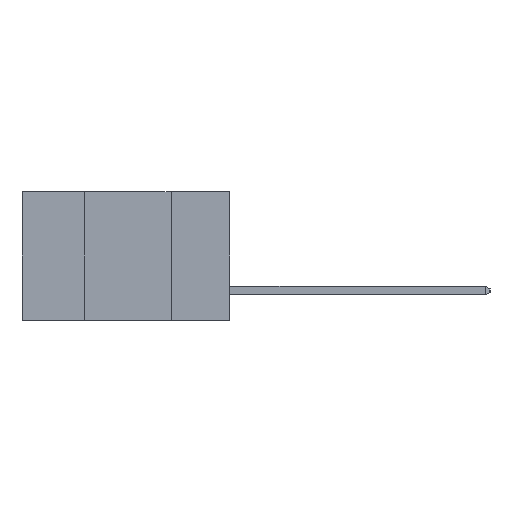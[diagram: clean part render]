
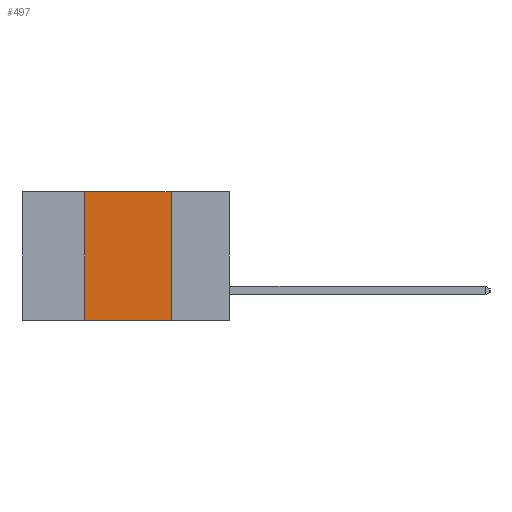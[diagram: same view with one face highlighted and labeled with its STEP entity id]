
A CAD part, left-side view. The second image highlights one B-rep face of the part: STEP entity #497.
In plain terms, the highlighted planar face has unit normal (-1, 0, 0).
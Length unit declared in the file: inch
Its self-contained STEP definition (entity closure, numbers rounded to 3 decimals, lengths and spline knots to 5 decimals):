
#38 = LINE ( 'NONE', #9414, #6349 ) ;
#82 = DIRECTION ( 'NONE',  ( 0., 0., -1. ) ) ;
#449 = CARTESIAN_POINT ( 'NONE',  ( 0., 0.6, 0. ) ) ;
#473 = CARTESIAN_POINT ( 'NONE',  ( 0., 0.42, 0. ) ) ;
#497 = ADVANCED_FACE ( 'NONE', ( #3796 ), #8172, .F. ) ;
#711 = DIRECTION ( 'NONE',  ( 0., 0., -1. ) ) ;
#1211 = EDGE_CURVE ( 'NONE', #5208, #2155, #4407, .T. ) ;
#1253 = LINE ( 'NONE', #449, #5254 ) ;
#1266 = EDGE_CURVE ( 'NONE', #5603, #5208, #1253, .T. ) ;
#1321 = EDGE_CURVE ( 'NONE', #3890, #2155, #38, .T. ) ;
#2155 = VERTEX_POINT ( 'NONE', #7296 ) ;
#2341 = ORIENTED_EDGE ( 'NONE', *, *, #8862, .F. ) ;
#2391 = CARTESIAN_POINT ( 'NONE',  ( 0., 0.42, -0.37 ) ) ;
#2506 = DIRECTION ( 'NONE',  ( 0., -1., 0. ) ) ;
#3792 = DIRECTION ( 'NONE',  ( 0., -1., 0. ) ) ;
#3796 = FACE_OUTER_BOUND ( 'NONE', #6502, .T. ) ;
#3890 = VERTEX_POINT ( 'NONE', #2391 ) ;
#4040 = ORIENTED_EDGE ( 'NONE', *, *, #1211, .F. ) ;
#4244 = LINE ( 'NONE', #5669, #9306 ) ;
#4407 = LINE ( 'NONE', #8159, #6482 ) ;
#4530 = DIRECTION ( 'NONE',  ( 1., 0., 0. ) ) ;
#5208 = VERTEX_POINT ( 'NONE', #7999 ) ;
#5254 = VECTOR ( 'NONE', #2506, 39.37008 ) ;
#5603 = VERTEX_POINT ( 'NONE', #473 ) ;
#5669 = CARTESIAN_POINT ( 'NONE',  ( 0., 0.42, -0.37 ) ) ;
#5997 = ORIENTED_EDGE ( 'NONE', *, *, #1266, .F. ) ;
#6349 = VECTOR ( 'NONE', #3792, 39.37008 ) ;
#6482 = VECTOR ( 'NONE', #711, 39.37008 ) ;
#6502 = EDGE_LOOP ( 'NONE', ( #4040, #5997, #2341, #7782 ) ) ;
#6699 = CARTESIAN_POINT ( 'NONE',  ( 0., 0.6, 0. ) ) ;
#6757 = AXIS2_PLACEMENT_3D ( 'NONE', #6699, #4530, #82 ) ;
#7296 = CARTESIAN_POINT ( 'NONE',  ( 0., 0.17, -0.37 ) ) ;
#7782 = ORIENTED_EDGE ( 'NONE', *, *, #1321, .T. ) ;
#7999 = CARTESIAN_POINT ( 'NONE',  ( 0., 0.17, 0. ) ) ;
#8159 = CARTESIAN_POINT ( 'NONE',  ( 0., 0.17, -0.37 ) ) ;
#8172 = PLANE ( 'NONE',  #6757 ) ;
#8862 = EDGE_CURVE ( 'NONE', #3890, #5603, #4244, .T. ) ;
#9306 = VECTOR ( 'NONE', #10111, 39.37008 ) ;
#9414 = CARTESIAN_POINT ( 'NONE',  ( 0., 0.6, -0.37 ) ) ;
#10111 = DIRECTION ( 'NONE',  ( 0., 0., 1. ) ) ;
